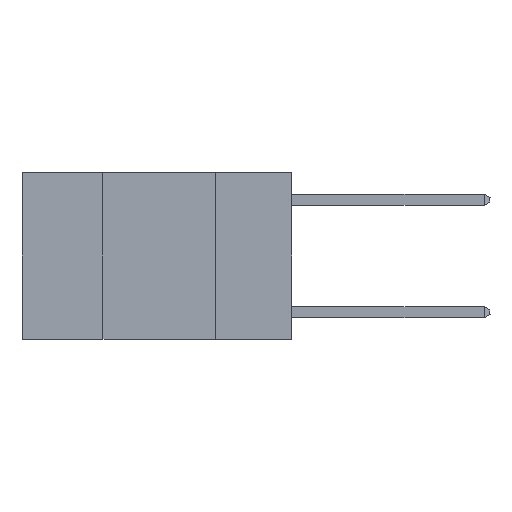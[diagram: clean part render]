
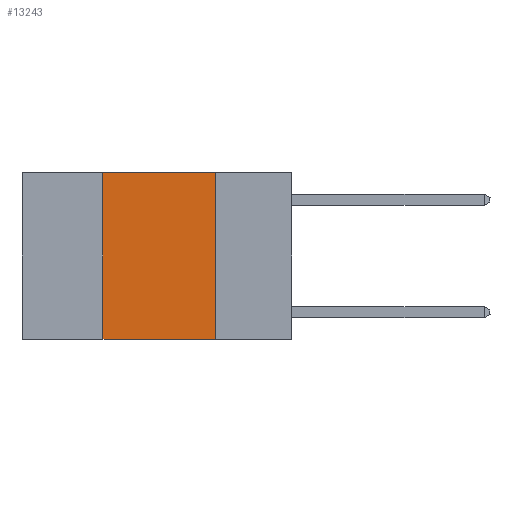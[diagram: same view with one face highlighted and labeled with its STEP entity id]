
A CAD part, left-side view. The second image highlights one B-rep face of the part: STEP entity #13243.
In plain terms, the highlighted planar face has unit normal (-1, 0, 0).
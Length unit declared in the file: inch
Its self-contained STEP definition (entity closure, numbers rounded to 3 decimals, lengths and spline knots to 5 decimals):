
#530 = CARTESIAN_POINT ( 'NONE',  ( 0., 0.17, -0.37 ) ) ;
#1181 = PLANE ( 'NONE',  #5372 ) ;
#1436 = CARTESIAN_POINT ( 'NONE',  ( 0., 0.17, 0. ) ) ;
#1568 = VECTOR ( 'NONE', #6162, 39.37008 ) ;
#2004 = CARTESIAN_POINT ( 'NONE',  ( 0., 0.42, 0. ) ) ;
#2007 = VECTOR ( 'NONE', #4930, 39.37008 ) ;
#2400 = DIRECTION ( 'NONE',  ( 1., 0., 0. ) ) ;
#2739 = VERTEX_POINT ( 'NONE', #7474 ) ;
#2853 = ORIENTED_EDGE ( 'NONE', *, *, #8050, .F. ) ;
#2946 = CARTESIAN_POINT ( 'NONE',  ( 0., 0.6, 0. ) ) ;
#3068 = DIRECTION ( 'NONE',  ( 0., 0., 1. ) ) ;
#3325 = EDGE_LOOP ( 'NONE', ( #2853, #5500, #8753, #12825 ) ) ;
#3850 = CARTESIAN_POINT ( 'NONE',  ( 0., 0.6, -0.37 ) ) ;
#4001 = EDGE_CURVE ( 'NONE', #9436, #14057, #9069, .T. ) ;
#4226 = EDGE_CURVE ( 'NONE', #2739, #10727, #11911, .T. ) ;
#4559 = DIRECTION ( 'NONE',  ( 0., 0., -1. ) ) ;
#4849 = FACE_OUTER_BOUND ( 'NONE', #3325, .T. ) ;
#4930 = DIRECTION ( 'NONE',  ( 0., -1., 0. ) ) ;
#5372 = AXIS2_PLACEMENT_3D ( 'NONE', #14968, #2400, #4559 ) ;
#5500 = ORIENTED_EDGE ( 'NONE', *, *, #4001, .F. ) ;
#5658 = VECTOR ( 'NONE', #12162, 39.37008 ) ;
#6162 = DIRECTION ( 'NONE',  ( 0., 0., -1. ) ) ;
#6228 = EDGE_CURVE ( 'NONE', #2739, #9436, #9868, .T. ) ;
#7474 = CARTESIAN_POINT ( 'NONE',  ( 0., 0.42, -0.37 ) ) ;
#7548 = CARTESIAN_POINT ( 'NONE',  ( 0., 0.17, 0. ) ) ;
#8050 = EDGE_CURVE ( 'NONE', #14057, #10727, #10792, .T. ) ;
#8753 = ORIENTED_EDGE ( 'NONE', *, *, #6228, .F. ) ;
#9069 = LINE ( 'NONE', #2946, #5658 ) ;
#9436 = VERTEX_POINT ( 'NONE', #10889 ) ;
#9468 = VECTOR ( 'NONE', #3068, 39.37008 ) ;
#9868 = LINE ( 'NONE', #2004, #9468 ) ;
#10727 = VERTEX_POINT ( 'NONE', #530 ) ;
#10792 = LINE ( 'NONE', #1436, #1568 ) ;
#10889 = CARTESIAN_POINT ( 'NONE',  ( 0., 0.42, 0. ) ) ;
#11911 = LINE ( 'NONE', #3850, #2007 ) ;
#12162 = DIRECTION ( 'NONE',  ( 0., -1., 0. ) ) ;
#12825 = ORIENTED_EDGE ( 'NONE', *, *, #4226, .T. ) ;
#13243 = ADVANCED_FACE ( 'NONE', ( #4849 ), #1181, .F. ) ;
#14057 = VERTEX_POINT ( 'NONE', #7548 ) ;
#14968 = CARTESIAN_POINT ( 'NONE',  ( 0., 0.6, 0. ) ) ;
